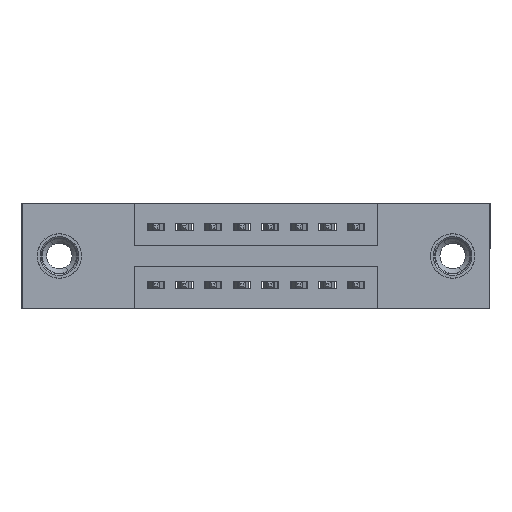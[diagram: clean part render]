
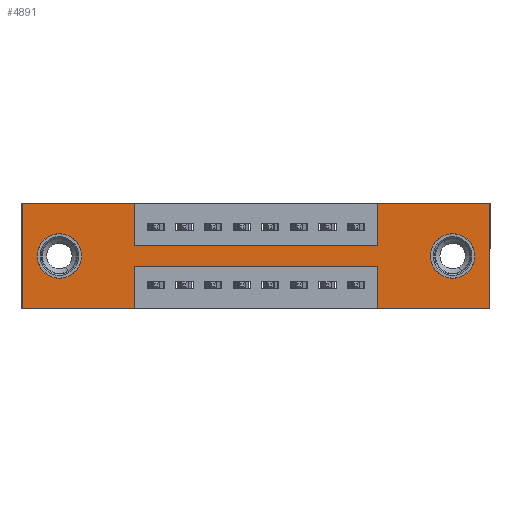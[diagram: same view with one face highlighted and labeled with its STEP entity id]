
A CAD part, front view. The second image highlights one B-rep face of the part: STEP entity #4891.
In plain terms, the highlighted planar face has unit normal (0, -1, 0).
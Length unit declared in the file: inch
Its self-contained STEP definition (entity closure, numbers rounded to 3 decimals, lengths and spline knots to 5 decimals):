
#10 = LINE ( 'NONE', #6328, #15314 ) ;
#46 = VERTEX_POINT ( 'NONE', #970 ) ;
#134 = CIRCLE ( 'NONE', #10150, 0.078 ) ;
#139 = LINE ( 'NONE', #6578, #14920 ) ;
#277 = CARTESIAN_POINT ( 'NONE',  ( 0.3925, 0., -0.15 ) ) ;
#407 = ORIENTED_EDGE ( 'NONE', *, *, #9371, .F. ) ;
#528 = CARTESIAN_POINT ( 'NONE',  ( 1.2425, 0., -0.37 ) ) ;
#547 = DIRECTION ( 'NONE',  ( 1., 0., 0. ) ) ;
#591 = ORIENTED_EDGE ( 'NONE', *, *, #1289, .F. ) ;
#604 = EDGE_LOOP ( 'NONE', ( #10339, #11201 ) ) ;
#622 = LINE ( 'NONE', #13537, #13094 ) ;
#637 = DIRECTION ( 'NONE',  ( 0., 0., -1. ) ) ;
#721 = CARTESIAN_POINT ( 'NONE',  ( 1.505, 0., -0.185 ) ) ;
#797 = DIRECTION ( 'NONE',  ( 0., 1., 0. ) ) ;
#962 = DIRECTION ( 'NONE',  ( 0., 0., -1. ) ) ;
#970 = CARTESIAN_POINT ( 'NONE',  ( 1.505, 0., -0.107 ) ) ;
#1070 = CARTESIAN_POINT ( 'NONE',  ( 1.2425, 0., 0. ) ) ;
#1115 = EDGE_CURVE ( 'NONE', #46, #13980, #7687, .T. ) ;
#1218 = DIRECTION ( 'NONE',  ( 0., 0., 1. ) ) ;
#1249 = CIRCLE ( 'NONE', #6810, 0.078 ) ;
#1289 = EDGE_CURVE ( 'NONE', #3570, #1676, #5786, .T. ) ;
#1344 = CARTESIAN_POINT ( 'NONE',  ( 1.2425, 0., -0.37 ) ) ;
#1355 = EDGE_CURVE ( 'NONE', #11623, #5291, #8696, .T. ) ;
#1676 = VERTEX_POINT ( 'NONE', #11652 ) ;
#1689 = VECTOR ( 'NONE', #1690, 39.37008 ) ;
#1690 = DIRECTION ( 'NONE',  ( 1., 0., 0. ) ) ;
#1924 = CARTESIAN_POINT ( 'NONE',  ( 0.3925, 0., 0. ) ) ;
#2095 = ORIENTED_EDGE ( 'NONE', *, *, #7111, .F. ) ;
#2118 = EDGE_CURVE ( 'NONE', #1676, #7883, #4877, .T. ) ;
#2452 = EDGE_CURVE ( 'NONE', #13980, #46, #6792, .T. ) ;
#2474 = EDGE_LOOP ( 'NONE', ( #2808, #11402 ) ) ;
#2520 = VECTOR ( 'NONE', #5872, 39.37008 ) ;
#2646 = VECTOR ( 'NONE', #637, 39.37008 ) ;
#2703 = VERTEX_POINT ( 'NONE', #14311 ) ;
#2761 = ORIENTED_EDGE ( 'NONE', *, *, #7369, .F. ) ;
#2808 = ORIENTED_EDGE ( 'NONE', *, *, #1115, .T. ) ;
#2926 = VERTEX_POINT ( 'NONE', #277 ) ;
#3114 = AXIS2_PLACEMENT_3D ( 'NONE', #721, #4048, #962 ) ;
#3119 = FACE_BOUND ( 'NONE', #2474, .T. ) ;
#3184 = ORIENTED_EDGE ( 'NONE', *, *, #1355, .F. ) ;
#3229 = DIRECTION ( 'NONE',  ( 0., -1., 0. ) ) ;
#3311 = VERTEX_POINT ( 'NONE', #3484 ) ;
#3484 = CARTESIAN_POINT ( 'NONE',  ( 1.635, 0., 0. ) ) ;
#3497 = AXIS2_PLACEMENT_3D ( 'NONE', #5243, #797, #9156 ) ;
#3570 = VERTEX_POINT ( 'NONE', #3936 ) ;
#3596 = ORIENTED_EDGE ( 'NONE', *, *, #14108, .F. ) ;
#3688 = CARTESIAN_POINT ( 'NONE',  ( 0., 0., -0.37 ) ) ;
#3691 = CARTESIAN_POINT ( 'NONE',  ( 1.2425, 0., -0.15 ) ) ;
#3936 = CARTESIAN_POINT ( 'NONE',  ( 0., 0., -0.37 ) ) ;
#4048 = DIRECTION ( 'NONE',  ( 0., 1., 0. ) ) ;
#4456 = ORIENTED_EDGE ( 'NONE', *, *, #2118, .F. ) ;
#4462 = CARTESIAN_POINT ( 'NONE',  ( 0., 0., -0.37 ) ) ;
#4591 = DIRECTION ( 'NONE',  ( -1., 0., 0. ) ) ;
#4605 = CARTESIAN_POINT ( 'NONE',  ( 0.3925, 0., -0.22 ) ) ;
#4808 = ORIENTED_EDGE ( 'NONE', *, *, #6210, .F. ) ;
#4877 = LINE ( 'NONE', #14326, #1689 ) ;
#4891 = ADVANCED_FACE ( 'NONE', ( #3119, #6324, #6715 ), #9262, .T. ) ;
#4975 = CARTESIAN_POINT ( 'NONE',  ( 0.13, 0., -0.107 ) ) ;
#5093 = DIRECTION ( 'NONE',  ( 1., 0., 0. ) ) ;
#5243 = CARTESIAN_POINT ( 'NONE',  ( 1.505, 0., -0.185 ) ) ;
#5291 = VERTEX_POINT ( 'NONE', #13498 ) ;
#5442 = DIRECTION ( 'NONE',  ( 0., 0., 1. ) ) ;
#5517 = DIRECTION ( 'NONE',  ( 0., 1., 0. ) ) ;
#5695 = DIRECTION ( 'NONE',  ( 0., 0., -1. ) ) ;
#5786 = LINE ( 'NONE', #11198, #12236 ) ;
#5854 = EDGE_CURVE ( 'NONE', #3311, #8326, #622, .T. ) ;
#5872 = DIRECTION ( 'NONE',  ( 0., 0., 1. ) ) ;
#5989 = VECTOR ( 'NONE', #11044, 39.37008 ) ;
#6210 = EDGE_CURVE ( 'NONE', #13227, #8312, #11793, .T. ) ;
#6224 = EDGE_LOOP ( 'NONE', ( #13682, #3184, #407, #12169, #11139, #2095, #4808, #3596, #6310, #4456, #591, #2761 ) ) ;
#6310 = ORIENTED_EDGE ( 'NONE', *, *, #14822, .F. ) ;
#6324 = FACE_BOUND ( 'NONE', #604, .T. ) ;
#6328 = CARTESIAN_POINT ( 'NONE',  ( 0., 0., 0. ) ) ;
#6578 = CARTESIAN_POINT ( 'NONE',  ( 0.3925, 0., -0.15 ) ) ;
#6607 = VERTEX_POINT ( 'NONE', #10280 ) ;
#6715 = FACE_OUTER_BOUND ( 'NONE', #6224, .T. ) ;
#6792 = CIRCLE ( 'NONE', #3114, 0.078 ) ;
#6810 = AXIS2_PLACEMENT_3D ( 'NONE', #7136, #8443, #1218 ) ;
#7111 = EDGE_CURVE ( 'NONE', #8312, #3311, #10, .T. ) ;
#7136 = CARTESIAN_POINT ( 'NONE',  ( 0.13, 0., -0.185 ) ) ;
#7369 = EDGE_CURVE ( 'NONE', #6607, #3570, #9316, .T. ) ;
#7516 = CARTESIAN_POINT ( 'NONE',  ( 0.3925, 0., -0.37 ) ) ;
#7687 = CIRCLE ( 'NONE', #3497, 0.078 ) ;
#7883 = VERTEX_POINT ( 'NONE', #1924 ) ;
#7971 = LINE ( 'NONE', #7516, #11237 ) ;
#8149 = CARTESIAN_POINT ( 'NONE',  ( 0., 0., -0.37 ) ) ;
#8312 = VERTEX_POINT ( 'NONE', #12424 ) ;
#8326 = VERTEX_POINT ( 'NONE', #10006 ) ;
#8443 = DIRECTION ( 'NONE',  ( 0., 1., 0. ) ) ;
#8696 = LINE ( 'NONE', #4605, #11935 ) ;
#9059 = EDGE_CURVE ( 'NONE', #2703, #9392, #134, .T. ) ;
#9065 = LINE ( 'NONE', #12730, #2646 ) ;
#9156 = DIRECTION ( 'NONE',  ( 0., 0., -1. ) ) ;
#9262 = PLANE ( 'NONE',  #11771 ) ;
#9316 = LINE ( 'NONE', #8149, #12155 ) ;
#9371 = EDGE_CURVE ( 'NONE', #14745, #11623, #12058, .T. ) ;
#9392 = VERTEX_POINT ( 'NONE', #4975 ) ;
#9662 = CARTESIAN_POINT ( 'NONE',  ( 1.2425, 0., -0.22 ) ) ;
#9680 = VECTOR ( 'NONE', #9785, 39.37008 ) ;
#9785 = DIRECTION ( 'NONE',  ( -1., 0., 0. ) ) ;
#9958 = EDGE_CURVE ( 'NONE', #9392, #2703, #1249, .T. ) ;
#10006 = CARTESIAN_POINT ( 'NONE',  ( 1.635, 0., -0.37 ) ) ;
#10072 = LINE ( 'NONE', #3688, #9680 ) ;
#10150 = AXIS2_PLACEMENT_3D ( 'NONE', #12750, #5517, #13965 ) ;
#10280 = CARTESIAN_POINT ( 'NONE',  ( 0.3925, 0., -0.37 ) ) ;
#10339 = ORIENTED_EDGE ( 'NONE', *, *, #9958, .T. ) ;
#10626 = DIRECTION ( 'NONE',  ( -1., 0., 0. ) ) ;
#11044 = DIRECTION ( 'NONE',  ( 0., 0., 1. ) ) ;
#11139 = ORIENTED_EDGE ( 'NONE', *, *, #5854, .F. ) ;
#11159 = CARTESIAN_POINT ( 'NONE',  ( 1.505, 0., -0.263 ) ) ;
#11198 = CARTESIAN_POINT ( 'NONE',  ( 0., 0., 0. ) ) ;
#11201 = ORIENTED_EDGE ( 'NONE', *, *, #9059, .T. ) ;
#11237 = VECTOR ( 'NONE', #14725, 39.37008 ) ;
#11402 = ORIENTED_EDGE ( 'NONE', *, *, #2452, .T. ) ;
#11623 = VERTEX_POINT ( 'NONE', #9662 ) ;
#11652 = CARTESIAN_POINT ( 'NONE',  ( 0., 0., 0. ) ) ;
#11771 = AXIS2_PLACEMENT_3D ( 'NONE', #4462, #3229, #5695 ) ;
#11793 = LINE ( 'NONE', #1070, #2520 ) ;
#11935 = VECTOR ( 'NONE', #4591, 39.37008 ) ;
#12058 = LINE ( 'NONE', #1344, #5989 ) ;
#12155 = VECTOR ( 'NONE', #10626, 39.37008 ) ;
#12169 = ORIENTED_EDGE ( 'NONE', *, *, #12865, .F. ) ;
#12236 = VECTOR ( 'NONE', #5442, 39.37008 ) ;
#12285 = EDGE_CURVE ( 'NONE', #5291, #6607, #7971, .T. ) ;
#12424 = CARTESIAN_POINT ( 'NONE',  ( 1.2425, 0., 0. ) ) ;
#12730 = CARTESIAN_POINT ( 'NONE',  ( 0.3925, 0., 0. ) ) ;
#12750 = CARTESIAN_POINT ( 'NONE',  ( 0.13, 0., -0.185 ) ) ;
#12865 = EDGE_CURVE ( 'NONE', #8326, #14745, #10072, .T. ) ;
#13094 = VECTOR ( 'NONE', #14740, 39.37008 ) ;
#13227 = VERTEX_POINT ( 'NONE', #3691 ) ;
#13498 = CARTESIAN_POINT ( 'NONE',  ( 0.3925, 0., -0.22 ) ) ;
#13537 = CARTESIAN_POINT ( 'NONE',  ( 1.635, 0., 0. ) ) ;
#13682 = ORIENTED_EDGE ( 'NONE', *, *, #12285, .F. ) ;
#13965 = DIRECTION ( 'NONE',  ( 0., 0., 1. ) ) ;
#13980 = VERTEX_POINT ( 'NONE', #11159 ) ;
#14108 = EDGE_CURVE ( 'NONE', #2926, #13227, #139, .T. ) ;
#14311 = CARTESIAN_POINT ( 'NONE',  ( 0.13, 0., -0.263 ) ) ;
#14326 = CARTESIAN_POINT ( 'NONE',  ( 0., 0., 0. ) ) ;
#14725 = DIRECTION ( 'NONE',  ( 0., 0., -1. ) ) ;
#14740 = DIRECTION ( 'NONE',  ( 0., 0., -1. ) ) ;
#14745 = VERTEX_POINT ( 'NONE', #528 ) ;
#14822 = EDGE_CURVE ( 'NONE', #7883, #2926, #9065, .T. ) ;
#14920 = VECTOR ( 'NONE', #547, 39.37008 ) ;
#15314 = VECTOR ( 'NONE', #5093, 39.37008 ) ;
